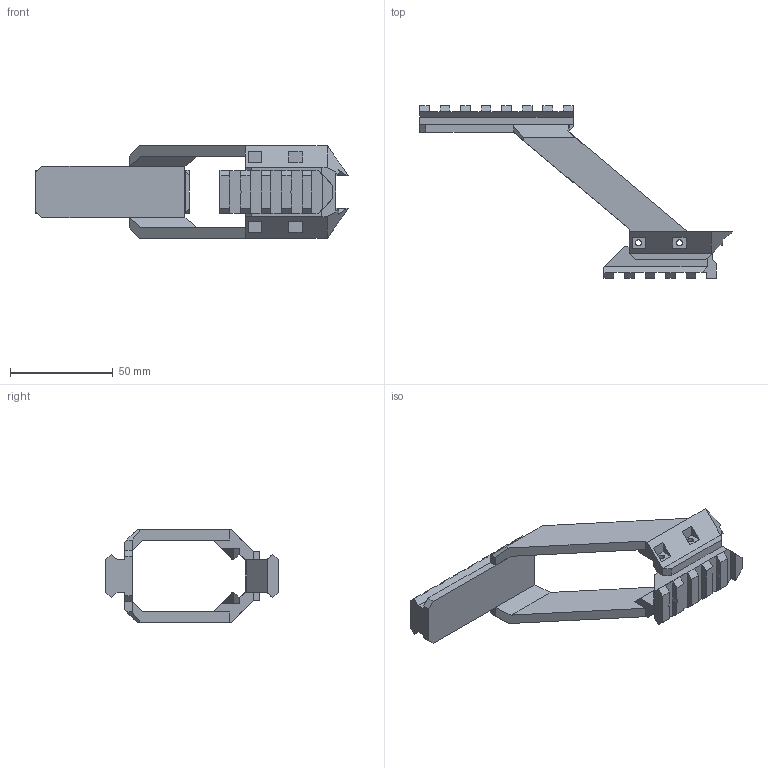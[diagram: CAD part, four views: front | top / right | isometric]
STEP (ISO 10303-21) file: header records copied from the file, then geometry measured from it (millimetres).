
FILE_DESCRIPTION(/* description */ (''),/* implementation_level */ '2;1');
FILE_NAME(/* name */ 'Big-Point Final_Sight Mount v1.step',/* time_stamp */ '2020-10-31T21:38:08-04:00',/* author */ (''),/* organization */ (''),/* preprocessor_version */ 'ST-DEVELOPER v18.1',/* originating_system */ 'Autodesk Translation Framework v9.3.0.1241',/* authorisation */ '');
FILE_SCHEMA (('AUTOMOTIVE_DESIGN { 1 0 10303 214 3 1 1 }'));
Length unit declared in the file: millimetre
Products named in the file (1): Big-Point Final_Sight Mount
Bounding box: 152.28 x 84 x 45.02 mm (x, y, z)
Volume: 52855.8 mm3; surface area: 22558.8 mm2
Topology: 1 solids, 1 shells, 211 faces, 619 edges, 408 vertices
Faces by surface type: plane 199, cylinder 12
Full cylindrical faces by diameter (mm): 3 x2
Entity records: 6926 total; most frequent: CARTESIAN_POINT 1239, ORIENTED_EDGE 1238, DIRECTION 1075, EDGE_CURVE 619, LINE 587, VECTOR 587, VERTEX_POINT 408, AXIS2_PLACEMENT_3D 244
